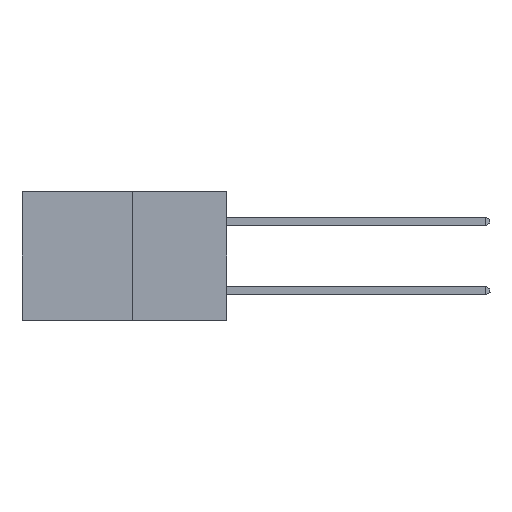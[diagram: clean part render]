
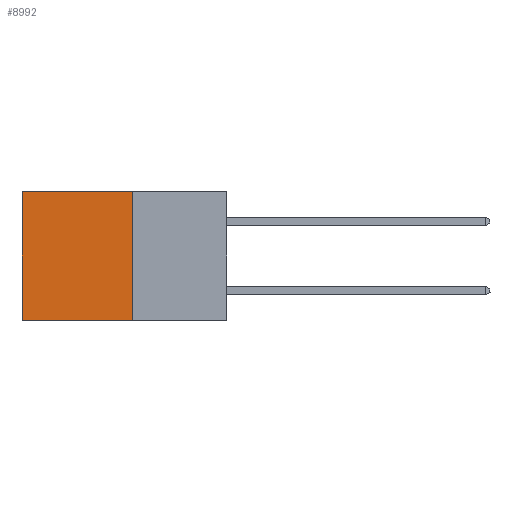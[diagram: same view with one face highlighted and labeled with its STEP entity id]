
A CAD part, left-side view. The second image highlights one B-rep face of the part: STEP entity #8992.
In plain terms, the highlighted planar face has unit normal (-1, 0, 0).
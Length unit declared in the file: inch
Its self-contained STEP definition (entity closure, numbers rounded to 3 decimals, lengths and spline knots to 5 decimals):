
#196 = EDGE_LOOP ( 'NONE', ( #3089, #5592, #5853, #2457 ) ) ;
#327 = DIRECTION ( 'NONE',  ( 0., 0., -1. ) ) ;
#441 = VERTEX_POINT ( 'NONE', #540 ) ;
#470 = VECTOR ( 'NONE', #2769, 39.37008 ) ;
#540 = CARTESIAN_POINT ( 'NONE',  ( 0.277, 0.27, 0. ) ) ;
#580 = VERTEX_POINT ( 'NONE', #4384 ) ;
#819 = PLANE ( 'NONE',  #8541 ) ;
#1737 = CARTESIAN_POINT ( 'NONE',  ( 0.277, 0.27, -0.37 ) ) ;
#2208 = LINE ( 'NONE', #3921, #7543 ) ;
#2317 = VECTOR ( 'NONE', #9538, 39.37008 ) ;
#2457 = ORIENTED_EDGE ( 'NONE', *, *, #5716, .T. ) ;
#2769 = DIRECTION ( 'NONE',  ( 0., 0., -1. ) ) ;
#3089 = ORIENTED_EDGE ( 'NONE', *, *, #5689, .T. ) ;
#3433 = DIRECTION ( 'NONE',  ( 0., 0., -1. ) ) ;
#3921 = CARTESIAN_POINT ( 'NONE',  ( 0.277, 0.27, -0.37 ) ) ;
#4007 = VECTOR ( 'NONE', #327, 39.37008 ) ;
#4384 = CARTESIAN_POINT ( 'NONE',  ( 0.277, 0.27, -0.37 ) ) ;
#4493 = CARTESIAN_POINT ( 'NONE',  ( 0.277, 0.27, 0. ) ) ;
#5211 = FACE_OUTER_BOUND ( 'NONE', #196, .T. ) ;
#5300 = CARTESIAN_POINT ( 'NONE',  ( 0.277, 0.59, -0.37 ) ) ;
#5592 = ORIENTED_EDGE ( 'NONE', *, *, #8719, .F. ) ;
#5689 = EDGE_CURVE ( 'NONE', #8156, #10940, #9267, .T. ) ;
#5716 = EDGE_CURVE ( 'NONE', #441, #8156, #9005, .T. ) ;
#5853 = ORIENTED_EDGE ( 'NONE', *, *, #9823, .F. ) ;
#6307 = CARTESIAN_POINT ( 'NONE',  ( 0.277, 0.27, -0.37 ) ) ;
#6890 = CARTESIAN_POINT ( 'NONE',  ( 0.277, 0.59, -0.37 ) ) ;
#7273 = DIRECTION ( 'NONE',  ( 0., 1., 0. ) ) ;
#7543 = VECTOR ( 'NONE', #7273, 39.37008 ) ;
#8156 = VERTEX_POINT ( 'NONE', #10844 ) ;
#8444 = DIRECTION ( 'NONE',  ( 1., 0., 0. ) ) ;
#8447 = LINE ( 'NONE', #6307, #4007 ) ;
#8541 = AXIS2_PLACEMENT_3D ( 'NONE', #1737, #8444, #3433 ) ;
#8719 = EDGE_CURVE ( 'NONE', #580, #10940, #2208, .T. ) ;
#8992 = ADVANCED_FACE ( 'NONE', ( #5211 ), #819, .F. ) ;
#9005 = LINE ( 'NONE', #4493, #2317 ) ;
#9267 = LINE ( 'NONE', #5300, #470 ) ;
#9538 = DIRECTION ( 'NONE',  ( 0., 1., 0. ) ) ;
#9823 = EDGE_CURVE ( 'NONE', #441, #580, #8447, .T. ) ;
#10844 = CARTESIAN_POINT ( 'NONE',  ( 0.277, 0.59, 0. ) ) ;
#10940 = VERTEX_POINT ( 'NONE', #6890 ) ;
